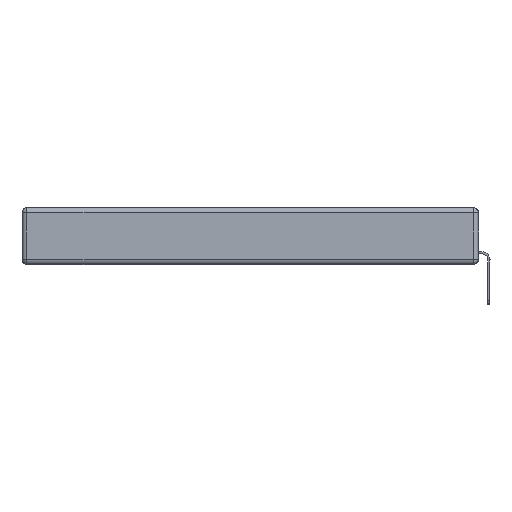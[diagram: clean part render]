
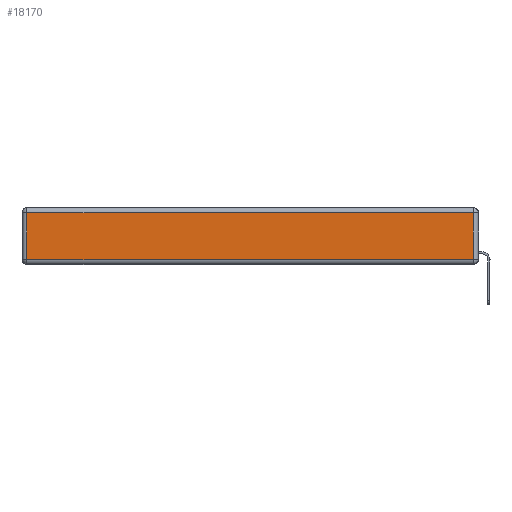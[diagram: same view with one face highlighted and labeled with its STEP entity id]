
A CAD part, left-side view. The second image highlights one B-rep face of the part: STEP entity #18170.
In plain terms, the highlighted planar face has unit normal (-1, 0, 0).
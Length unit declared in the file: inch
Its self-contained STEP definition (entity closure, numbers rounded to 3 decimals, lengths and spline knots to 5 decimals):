
#640 = EDGE_CURVE ( 'NONE', #9886, #6453, #19126, .T. ) ;
#1351 = VECTOR ( 'NONE', #9410, 39.37008 ) ;
#1357 = CARTESIAN_POINT ( 'NONE',  ( 0., 0., -0.313 ) ) ;
#1760 = CARTESIAN_POINT ( 'NONE',  ( 0., 0.03, -0.03 ) ) ;
#1766 = LINE ( 'NONE', #21627, #8161 ) ;
#2107 = CARTESIAN_POINT ( 'NONE',  ( 0., 2.72, -0.03 ) ) ;
#2287 = CARTESIAN_POINT ( 'NONE',  ( 0., 2.72, -0.313 ) ) ;
#2356 = CARTESIAN_POINT ( 'NONE',  ( 0., 0.03, -0.343 ) ) ;
#3894 = CARTESIAN_POINT ( 'NONE',  ( 0., 0., -0.343 ) ) ;
#4028 = DIRECTION ( 'NONE',  ( 0., 0., 1. ) ) ;
#4303 = DIRECTION ( 'NONE',  ( 0., 0., 1. ) ) ;
#6109 = DIRECTION ( 'NONE',  ( -1., 0., 0. ) ) ;
#6453 = VERTEX_POINT ( 'NONE', #2287 ) ;
#6658 = EDGE_CURVE ( 'NONE', #6453, #9072, #17083, .T. ) ;
#6694 = AXIS2_PLACEMENT_3D ( 'NONE', #3894, #6109, #4028 ) ;
#6964 = ORIENTED_EDGE ( 'NONE', *, *, #6658, .T. ) ;
#8048 = FACE_OUTER_BOUND ( 'NONE', #12900, .T. ) ;
#8161 = VECTOR ( 'NONE', #9968, 39.37008 ) ;
#8506 = ORIENTED_EDGE ( 'NONE', *, *, #640, .T. ) ;
#9072 = VERTEX_POINT ( 'NONE', #14517 ) ;
#9410 = DIRECTION ( 'NONE',  ( 0., 0., -1. ) ) ;
#9886 = VERTEX_POINT ( 'NONE', #2107 ) ;
#9968 = DIRECTION ( 'NONE',  ( 0., 1., 0. ) ) ;
#10437 = ORIENTED_EDGE ( 'NONE', *, *, #10667, .T. ) ;
#10548 = VECTOR ( 'NONE', #21107, 39.37008 ) ;
#10667 = EDGE_CURVE ( 'NONE', #20421, #9886, #1766, .T. ) ;
#11766 = ORIENTED_EDGE ( 'NONE', *, *, #19626, .T. ) ;
#12900 = EDGE_LOOP ( 'NONE', ( #6964, #11766, #10437, #8506 ) ) ;
#13041 = CARTESIAN_POINT ( 'NONE',  ( 0., 2.72, -0.343 ) ) ;
#14517 = CARTESIAN_POINT ( 'NONE',  ( 0., 0.03, -0.313 ) ) ;
#17083 = LINE ( 'NONE', #1357, #10548 ) ;
#17831 = LINE ( 'NONE', #2356, #18692 ) ;
#18170 = ADVANCED_FACE ( 'NONE', ( #8048 ), #21791, .T. ) ;
#18692 = VECTOR ( 'NONE', #4303, 39.37008 ) ;
#19126 = LINE ( 'NONE', #13041, #1351 ) ;
#19626 = EDGE_CURVE ( 'NONE', #9072, #20421, #17831, .T. ) ;
#20421 = VERTEX_POINT ( 'NONE', #1760 ) ;
#21107 = DIRECTION ( 'NONE',  ( 0., -1., 0. ) ) ;
#21627 = CARTESIAN_POINT ( 'NONE',  ( 0., 2.75, -0.03 ) ) ;
#21791 = PLANE ( 'NONE',  #6694 ) ;
